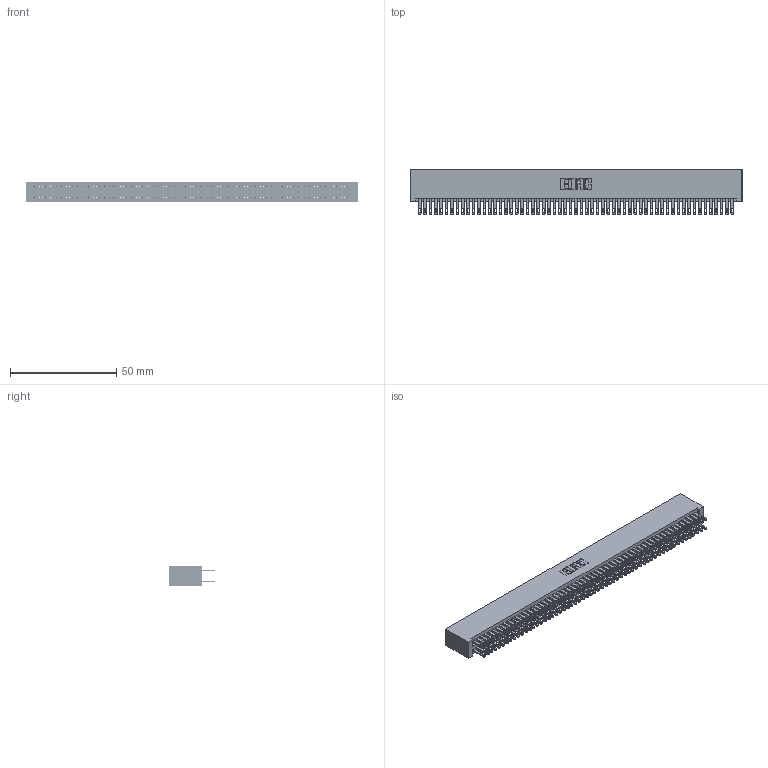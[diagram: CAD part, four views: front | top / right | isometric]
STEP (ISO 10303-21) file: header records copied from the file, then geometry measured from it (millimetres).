
FILE_DESCRIPTION (( 'STEP AP203' ), '1' );
FILE_NAME ('345-118-500-201.STEP', '2018-10-18T20:42:56', ( '' ), ( '' ), 'SwSTEP 2.0', 'SolidWorks 2016', '' );
FILE_SCHEMA (( 'CONFIG_CONTROL_DESIGN' ));
Length unit declared in the file: inch
Products named in the file (3): 345-118-500-201; 345 Part_No Mounting Lugs; 345-292-001_345-293-100
Assembly tree (119 placements, depth 2):
  345-118-500-201
    345 Part_No Mounting Lugs
    345-292-001_345-293-100  x118
Bounding box: 156.46 x 21.51 x 9.4 mm (x, y, z)
Volume: 16333.4 mm3; surface area: 25979.5 mm2
Topology: 119 solids, 119 shells, 5546 faces, 16955 edges, 11302 vertices
Faces by surface type: plane 3262, cylinder 2284
Entity records: 43657 total; most frequent: CARTESIAN_POINT 7300, ORIENTED_EDGE 7234, DIRECTION 6413, EDGE_CURVE 3617, VECTOR 3253, LINE 3253, VERTEX_POINT 2410, AXIS2_PLACEMENT_3D 1580
